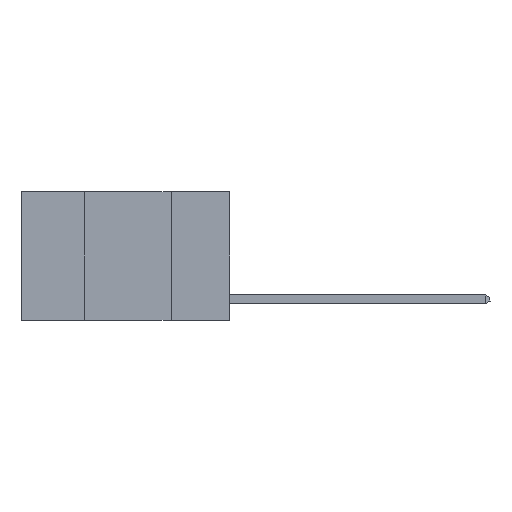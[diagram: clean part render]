
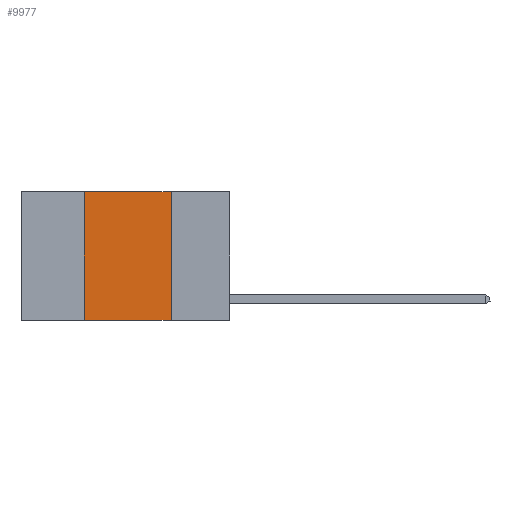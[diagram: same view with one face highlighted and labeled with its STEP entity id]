
A CAD part, left-side view. The second image highlights one B-rep face of the part: STEP entity #9977.
In plain terms, the highlighted planar face has unit normal (-1, 0, 0).
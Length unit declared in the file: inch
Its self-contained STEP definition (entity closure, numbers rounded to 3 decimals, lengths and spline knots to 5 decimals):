
#17 = CARTESIAN_POINT ( 'NONE',  ( 0., 0.6, 0. ) ) ;
#1484 = DIRECTION ( 'NONE',  ( 1., 0., 0. ) ) ;
#1698 = CARTESIAN_POINT ( 'NONE',  ( 0., 0.17, 0. ) ) ;
#2422 = CARTESIAN_POINT ( 'NONE',  ( 0., 0.17, 0. ) ) ;
#2738 = EDGE_CURVE ( 'NONE', #6097, #11161, #11846, .T. ) ;
#2892 = ORIENTED_EDGE ( 'NONE', *, *, #2738, .F. ) ;
#3198 = DIRECTION ( 'NONE',  ( 0., 0., -1. ) ) ;
#3507 = CARTESIAN_POINT ( 'NONE',  ( 0., 0.17, -0.37 ) ) ;
#3782 = LINE ( 'NONE', #10753, #17409 ) ;
#3800 = CARTESIAN_POINT ( 'NONE',  ( 0., 0.42, 0. ) ) ;
#3872 = DIRECTION ( 'NONE',  ( 0., 0., 1. ) ) ;
#4860 = DIRECTION ( 'NONE',  ( 0., -1., 0. ) ) ;
#5686 = VERTEX_POINT ( 'NONE', #6497 ) ;
#6097 = VERTEX_POINT ( 'NONE', #3800 ) ;
#6157 = VERTEX_POINT ( 'NONE', #3507 ) ;
#6251 = CARTESIAN_POINT ( 'NONE',  ( 0., 0.6, 0. ) ) ;
#6497 = CARTESIAN_POINT ( 'NONE',  ( 0., 0.42, -0.37 ) ) ;
#7900 = EDGE_CURVE ( 'NONE', #5686, #6157, #15761, .T. ) ;
#8245 = VECTOR ( 'NONE', #10674, 39.37008 ) ;
#8802 = VECTOR ( 'NONE', #4860, 39.37008 ) ;
#8952 = CARTESIAN_POINT ( 'NONE',  ( 0., 0.6, -0.37 ) ) ;
#9737 = EDGE_CURVE ( 'NONE', #5686, #6097, #3782, .T. ) ;
#9977 = ADVANCED_FACE ( 'NONE', ( #14405 ), #16328, .F. ) ;
#10674 = DIRECTION ( 'NONE',  ( 0., -1., 0. ) ) ;
#10753 = CARTESIAN_POINT ( 'NONE',  ( 0., 0.42, 0. ) ) ;
#10798 = ORIENTED_EDGE ( 'NONE', *, *, #9737, .F. ) ;
#10861 = VECTOR ( 'NONE', #3198, 39.37008 ) ;
#11161 = VERTEX_POINT ( 'NONE', #2422 ) ;
#11264 = DIRECTION ( 'NONE',  ( 0., 0., -1. ) ) ;
#11532 = EDGE_CURVE ( 'NONE', #11161, #6157, #13973, .T. ) ;
#11846 = LINE ( 'NONE', #6251, #8245 ) ;
#12075 = ORIENTED_EDGE ( 'NONE', *, *, #7900, .T. ) ;
#13973 = LINE ( 'NONE', #1698, #10861 ) ;
#14405 = FACE_OUTER_BOUND ( 'NONE', #17220, .T. ) ;
#15289 = ORIENTED_EDGE ( 'NONE', *, *, #11532, .F. ) ;
#15659 = AXIS2_PLACEMENT_3D ( 'NONE', #17, #1484, #11264 ) ;
#15761 = LINE ( 'NONE', #8952, #8802 ) ;
#16328 = PLANE ( 'NONE',  #15659 ) ;
#17220 = EDGE_LOOP ( 'NONE', ( #15289, #2892, #10798, #12075 ) ) ;
#17409 = VECTOR ( 'NONE', #3872, 39.37008 ) ;
